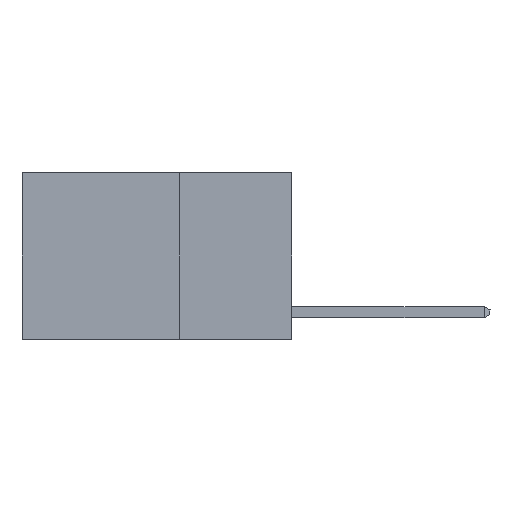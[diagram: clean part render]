
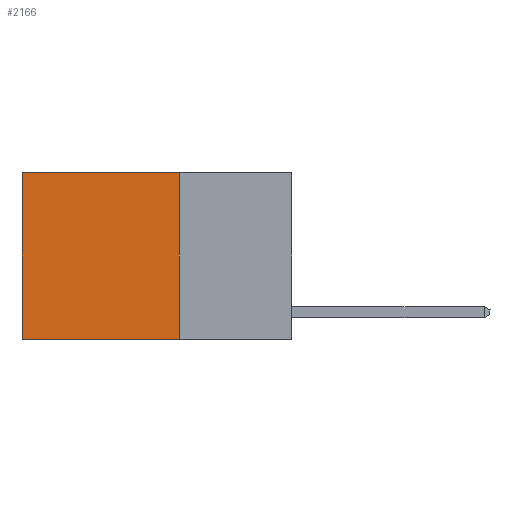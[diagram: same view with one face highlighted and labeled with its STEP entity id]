
A CAD part, left-side view. The second image highlights one B-rep face of the part: STEP entity #2166.
In plain terms, the highlighted planar face has unit normal (-1, 0, 0).
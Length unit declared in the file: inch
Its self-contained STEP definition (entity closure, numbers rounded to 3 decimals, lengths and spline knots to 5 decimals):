
#318 = EDGE_CURVE ( 'NONE', #6354, #5608, #2150, .T. ) ;
#349 = PLANE ( 'NONE',  #4064 ) ;
#407 = DIRECTION ( 'NONE',  ( 1., 0., 0. ) ) ;
#409 = VERTEX_POINT ( 'NONE', #5868 ) ;
#2150 = LINE ( 'NONE', #8338, #4042 ) ;
#2166 = ADVANCED_FACE ( 'NONE', ( #15364 ), #349, .F. ) ;
#2325 = VERTEX_POINT ( 'NONE', #15664 ) ;
#2678 = DIRECTION ( 'NONE',  ( 0., 1., 0. ) ) ;
#4042 = VECTOR ( 'NONE', #13841, 39.37008 ) ;
#4064 = AXIS2_PLACEMENT_3D ( 'NONE', #13758, #407, #5739 ) ;
#4361 = LINE ( 'NONE', #10293, #10889 ) ;
#4398 = DIRECTION ( 'NONE',  ( 0., 1., 0. ) ) ;
#5439 = CARTESIAN_POINT ( 'NONE',  ( 0.2625, 0.25, -0.37 ) ) ;
#5494 = CARTESIAN_POINT ( 'NONE',  ( 0.2625, 0.25, 0. ) ) ;
#5608 = VERTEX_POINT ( 'NONE', #7621 ) ;
#5739 = DIRECTION ( 'NONE',  ( 0., 0., -1. ) ) ;
#5776 = VECTOR ( 'NONE', #2678, 39.37008 ) ;
#5868 = CARTESIAN_POINT ( 'NONE',  ( 0.2625, 0.25, 0. ) ) ;
#6354 = VERTEX_POINT ( 'NONE', #15415 ) ;
#6735 = EDGE_CURVE ( 'NONE', #2325, #5608, #11063, .T. ) ;
#6757 = ORIENTED_EDGE ( 'NONE', *, *, #8263, .T. ) ;
#7621 = CARTESIAN_POINT ( 'NONE',  ( 0.2625, 0.6, -0.37 ) ) ;
#8263 = EDGE_CURVE ( 'NONE', #409, #6354, #11875, .T. ) ;
#8338 = CARTESIAN_POINT ( 'NONE',  ( 0.2625, 0.6, 0. ) ) ;
#8670 = ORIENTED_EDGE ( 'NONE', *, *, #13994, .F. ) ;
#9473 = EDGE_LOOP ( 'NONE', ( #15314, #12136, #8670, #6757 ) ) ;
#10293 = CARTESIAN_POINT ( 'NONE',  ( 0.2625, 0.25, 0. ) ) ;
#10889 = VECTOR ( 'NONE', #16957, 39.37008 ) ;
#11063 = LINE ( 'NONE', #5439, #17309 ) ;
#11875 = LINE ( 'NONE', #5494, #5776 ) ;
#12136 = ORIENTED_EDGE ( 'NONE', *, *, #6735, .F. ) ;
#13758 = CARTESIAN_POINT ( 'NONE',  ( 0.2625, 0.25, 0. ) ) ;
#13841 = DIRECTION ( 'NONE',  ( 0., 0., -1. ) ) ;
#13994 = EDGE_CURVE ( 'NONE', #409, #2325, #4361, .T. ) ;
#15314 = ORIENTED_EDGE ( 'NONE', *, *, #318, .T. ) ;
#15364 = FACE_OUTER_BOUND ( 'NONE', #9473, .T. ) ;
#15415 = CARTESIAN_POINT ( 'NONE',  ( 0.2625, 0.6, 0. ) ) ;
#15664 = CARTESIAN_POINT ( 'NONE',  ( 0.2625, 0.25, -0.37 ) ) ;
#16957 = DIRECTION ( 'NONE',  ( 0., 0., -1. ) ) ;
#17309 = VECTOR ( 'NONE', #4398, 39.37008 ) ;
